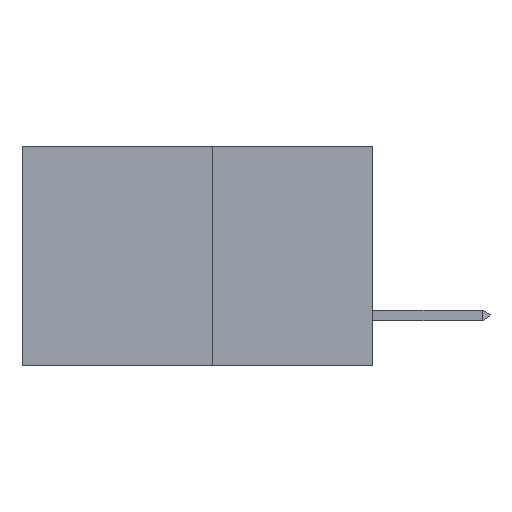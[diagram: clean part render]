
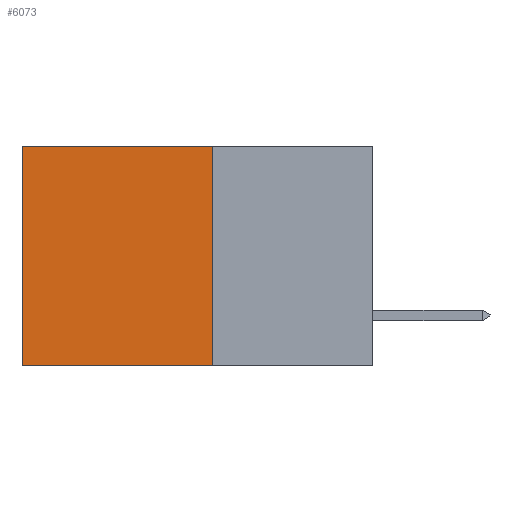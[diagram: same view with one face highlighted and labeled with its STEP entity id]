
A CAD part, left-side view. The second image highlights one B-rep face of the part: STEP entity #6073.
In plain terms, the highlighted planar face has unit normal (-1, 0, 0).
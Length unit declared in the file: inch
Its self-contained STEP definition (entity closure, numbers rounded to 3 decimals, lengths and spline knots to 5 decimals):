
#85 = CARTESIAN_POINT ( 'NONE',  ( 0.277, 0.27, 0. ) ) ;
#96 = VECTOR ( 'NONE', #10483, 39.37008 ) ;
#671 = CARTESIAN_POINT ( 'NONE',  ( 0.277, 0.27, -0.37 ) ) ;
#900 = ORIENTED_EDGE ( 'NONE', *, *, #3831, .T. ) ;
#2018 = CARTESIAN_POINT ( 'NONE',  ( 0.277, 0.59, -0.37 ) ) ;
#2022 = VECTOR ( 'NONE', #10654, 39.37008 ) ;
#2293 = LINE ( 'NONE', #9097, #9513 ) ;
#2915 = EDGE_CURVE ( 'NONE', #3442, #11823, #9563, .T. ) ;
#2974 = LINE ( 'NONE', #10663, #96 ) ;
#3442 = VERTEX_POINT ( 'NONE', #10253 ) ;
#3831 = EDGE_CURVE ( 'NONE', #9077, #4212, #2974, .T. ) ;
#4212 = VERTEX_POINT ( 'NONE', #4804 ) ;
#4804 = CARTESIAN_POINT ( 'NONE',  ( 0.277, 0.59, 0. ) ) ;
#5601 = EDGE_CURVE ( 'NONE', #4212, #11823, #12260, .T. ) ;
#5923 = ORIENTED_EDGE ( 'NONE', *, *, #5601, .T. ) ;
#6073 = ADVANCED_FACE ( 'NONE', ( #7501 ), #6194, .F. ) ;
#6156 = DIRECTION ( 'NONE',  ( 0., 0., -1. ) ) ;
#6171 = DIRECTION ( 'NONE',  ( 1., 0., 0. ) ) ;
#6194 = PLANE ( 'NONE',  #9197 ) ;
#6305 = CARTESIAN_POINT ( 'NONE',  ( 0.277, 0.27, -0.37 ) ) ;
#7501 = FACE_OUTER_BOUND ( 'NONE', #9262, .T. ) ;
#8350 = ORIENTED_EDGE ( 'NONE', *, *, #2915, .F. ) ;
#9077 = VERTEX_POINT ( 'NONE', #85 ) ;
#9097 = CARTESIAN_POINT ( 'NONE',  ( 0.277, 0.27, -0.37 ) ) ;
#9197 = AXIS2_PLACEMENT_3D ( 'NONE', #6305, #6171, #6156 ) ;
#9262 = EDGE_LOOP ( 'NONE', ( #5923, #8350, #10692, #900 ) ) ;
#9322 = EDGE_CURVE ( 'NONE', #9077, #3442, #2293, .T. ) ;
#9399 = VECTOR ( 'NONE', #9497, 39.37008 ) ;
#9497 = DIRECTION ( 'NONE',  ( 0., 0., -1. ) ) ;
#9513 = VECTOR ( 'NONE', #10223, 39.37008 ) ;
#9552 = CARTESIAN_POINT ( 'NONE',  ( 0.277, 0.59, -0.37 ) ) ;
#9563 = LINE ( 'NONE', #671, #2022 ) ;
#10223 = DIRECTION ( 'NONE',  ( 0., 0., -1. ) ) ;
#10253 = CARTESIAN_POINT ( 'NONE',  ( 0.277, 0.27, -0.37 ) ) ;
#10483 = DIRECTION ( 'NONE',  ( 0., 1., 0. ) ) ;
#10654 = DIRECTION ( 'NONE',  ( 0., 1., 0. ) ) ;
#10663 = CARTESIAN_POINT ( 'NONE',  ( 0.277, 0.27, 0. ) ) ;
#10692 = ORIENTED_EDGE ( 'NONE', *, *, #9322, .F. ) ;
#11823 = VERTEX_POINT ( 'NONE', #2018 ) ;
#12260 = LINE ( 'NONE', #9552, #9399 ) ;
